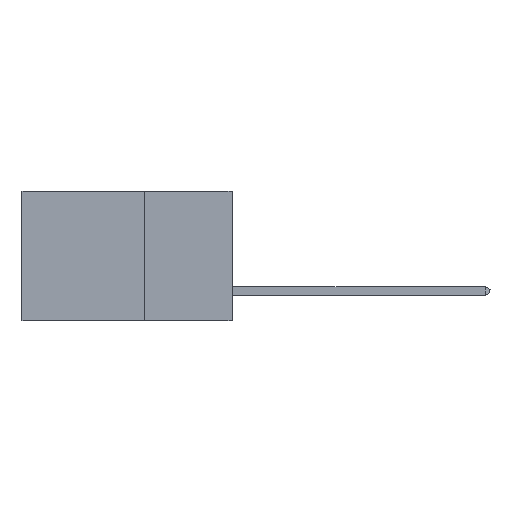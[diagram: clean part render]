
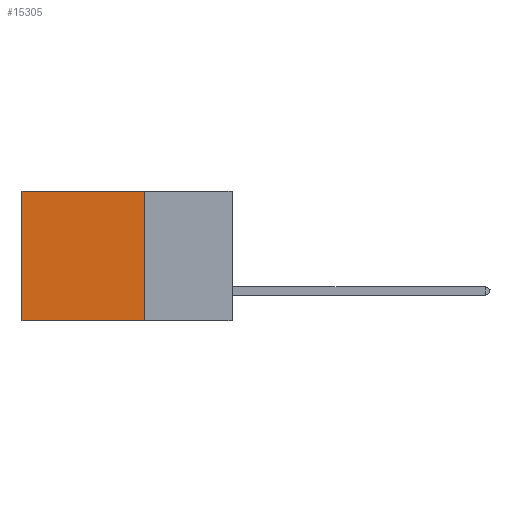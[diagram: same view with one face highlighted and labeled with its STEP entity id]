
A CAD part, left-side view. The second image highlights one B-rep face of the part: STEP entity #15305.
In plain terms, the highlighted planar face has unit normal (-1, 0, 0).
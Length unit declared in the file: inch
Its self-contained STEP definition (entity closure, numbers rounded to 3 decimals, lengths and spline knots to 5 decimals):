
#613 = EDGE_CURVE ( 'NONE', #42083, #14334, #46673, .T. ) ;
#1124 = CARTESIAN_POINT ( 'NONE',  ( 0.2875, 0.25, 0. ) ) ;
#3675 = ORIENTED_EDGE ( 'NONE', *, *, #15688, .F. ) ;
#4516 = DIRECTION ( 'NONE',  ( 0., 0., -1. ) ) ;
#6375 = VERTEX_POINT ( 'NONE', #13760 ) ;
#7002 = DIRECTION ( 'NONE',  ( 0., 1., 0. ) ) ;
#7522 = ORIENTED_EDGE ( 'NONE', *, *, #19658, .F. ) ;
#10120 = CARTESIAN_POINT ( 'NONE',  ( 0.2875, 0.25, 0. ) ) ;
#10910 = LINE ( 'NONE', #1124, #27055 ) ;
#13760 = CARTESIAN_POINT ( 'NONE',  ( 0.2875, 0.6, -0.37 ) ) ;
#14334 = VERTEX_POINT ( 'NONE', #32794 ) ;
#14522 = EDGE_LOOP ( 'NONE', ( #25219, #7522, #3675, #37898 ) ) ;
#15305 = ADVANCED_FACE ( 'NONE', ( #35278 ), #17762, .F. ) ;
#15688 = EDGE_CURVE ( 'NONE', #42083, #41542, #10910, .T. ) ;
#16245 = VECTOR ( 'NONE', #4516, 39.37008 ) ;
#16544 = LINE ( 'NONE', #39691, #24782 ) ;
#17762 = PLANE ( 'NONE',  #19524 ) ;
#19391 = CARTESIAN_POINT ( 'NONE',  ( 0.2875, 0.6, 0. ) ) ;
#19524 = AXIS2_PLACEMENT_3D ( 'NONE', #21544, #43790, #25268 ) ;
#19658 = EDGE_CURVE ( 'NONE', #41542, #6375, #16544, .T. ) ;
#21544 = CARTESIAN_POINT ( 'NONE',  ( 0.2875, 0.25, 0. ) ) ;
#24782 = VECTOR ( 'NONE', #31998, 39.37008 ) ;
#25219 = ORIENTED_EDGE ( 'NONE', *, *, #25927, .T. ) ;
#25268 = DIRECTION ( 'NONE',  ( 0., 0., -1. ) ) ;
#25927 = EDGE_CURVE ( 'NONE', #14334, #6375, #40780, .T. ) ;
#27055 = VECTOR ( 'NONE', #42008, 39.37008 ) ;
#31998 = DIRECTION ( 'NONE',  ( 0., 1., 0. ) ) ;
#32794 = CARTESIAN_POINT ( 'NONE',  ( 0.2875, 0.6, 0. ) ) ;
#33140 = CARTESIAN_POINT ( 'NONE',  ( 0.2875, 0.25, -0.37 ) ) ;
#35278 = FACE_OUTER_BOUND ( 'NONE', #14522, .T. ) ;
#37898 = ORIENTED_EDGE ( 'NONE', *, *, #613, .T. ) ;
#39691 = CARTESIAN_POINT ( 'NONE',  ( 0.2875, 0.25, -0.37 ) ) ;
#40780 = LINE ( 'NONE', #19391, #16245 ) ;
#41542 = VERTEX_POINT ( 'NONE', #33140 ) ;
#42008 = DIRECTION ( 'NONE',  ( 0., 0., -1. ) ) ;
#42083 = VERTEX_POINT ( 'NONE', #10120 ) ;
#42602 = VECTOR ( 'NONE', #7002, 39.37008 ) ;
#43633 = CARTESIAN_POINT ( 'NONE',  ( 0.2875, 0.25, 0. ) ) ;
#43790 = DIRECTION ( 'NONE',  ( 1., 0., 0. ) ) ;
#46673 = LINE ( 'NONE', #43633, #42602 ) ;
